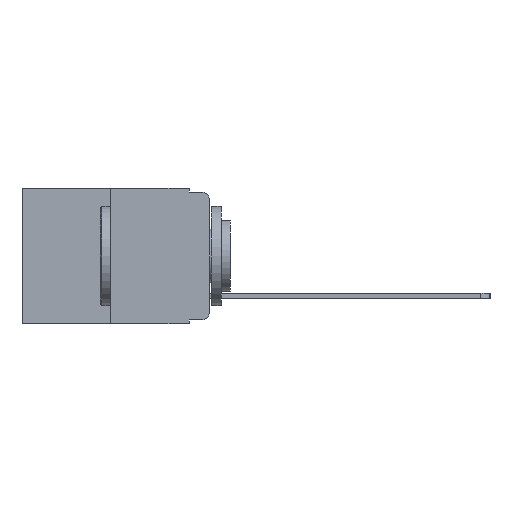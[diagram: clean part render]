
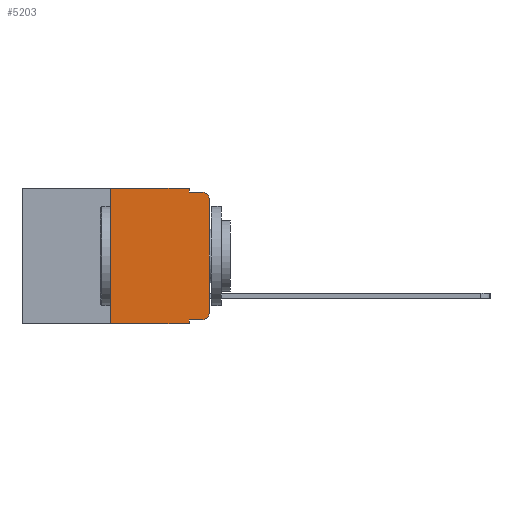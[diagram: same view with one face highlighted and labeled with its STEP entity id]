
A CAD part, left-side view. The second image highlights one B-rep face of the part: STEP entity #5203.
In plain terms, the highlighted planar face has unit normal (-1, 0, 0).
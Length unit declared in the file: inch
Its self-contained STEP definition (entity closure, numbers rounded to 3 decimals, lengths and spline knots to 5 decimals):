
#146 = LINE ( 'NONE', #504, #11594 ) ;
#258 = VERTEX_POINT ( 'NONE', #9818 ) ;
#504 = CARTESIAN_POINT ( 'NONE',  ( 0., 0., 0. ) ) ;
#538 = ORIENTED_EDGE ( 'NONE', *, *, #5592, .F. ) ;
#707 = ORIENTED_EDGE ( 'NONE', *, *, #5393, .F. ) ;
#801 = CARTESIAN_POINT ( 'NONE',  ( 0., 0.051, 0. ) ) ;
#826 = EDGE_CURVE ( 'NONE', #8402, #5616, #2717, .T. ) ;
#912 = ORIENTED_EDGE ( 'NONE', *, *, #3249, .F. ) ;
#1109 = VECTOR ( 'NONE', #1333, 39.37008 ) ;
#1115 = LINE ( 'NONE', #12775, #3952 ) ;
#1333 = DIRECTION ( 'NONE',  ( 0., 0., -1. ) ) ;
#1358 = CARTESIAN_POINT ( 'NONE',  ( 0., 0.051, 0. ) ) ;
#1480 = VERTEX_POINT ( 'NONE', #3114 ) ;
#1545 = VERTEX_POINT ( 'NONE', #9407 ) ;
#1655 = EDGE_CURVE ( 'NONE', #8402, #1545, #4308, .T. ) ;
#1674 = LINE ( 'NONE', #5324, #12825 ) ;
#1754 = ORIENTED_EDGE ( 'NONE', *, *, #10000, .T. ) ;
#1782 = ORIENTED_EDGE ( 'NONE', *, *, #9841, .T. ) ;
#1915 = ORIENTED_EDGE ( 'NONE', *, *, #7054, .T. ) ;
#2150 = CARTESIAN_POINT ( 'NONE',  ( 0., 0.051, 0. ) ) ;
#2279 = ORIENTED_EDGE ( 'NONE', *, *, #1655, .F. ) ;
#2567 = DIRECTION ( 'NONE',  ( -1., 0., 0. ) ) ;
#2634 = ORIENTED_EDGE ( 'NONE', *, *, #826, .T. ) ;
#2717 = LINE ( 'NONE', #13334, #13717 ) ;
#2757 = FACE_OUTER_BOUND ( 'NONE', #4951, .T. ) ;
#3110 = LINE ( 'NONE', #801, #14028 ) ;
#3114 = CARTESIAN_POINT ( 'NONE',  ( 0., 0.25, -0.343 ) ) ;
#3249 = EDGE_CURVE ( 'NONE', #1480, #258, #1674, .T. ) ;
#3304 = LINE ( 'NONE', #12474, #8816 ) ;
#3351 = ORIENTED_EDGE ( 'NONE', *, *, #13469, .T. ) ;
#3540 = DIRECTION ( 'NONE',  ( 0., 0., 1. ) ) ;
#3573 = DIRECTION ( 'NONE',  ( 0., -1., 0. ) ) ;
#3952 = VECTOR ( 'NONE', #10757, 39.37008 ) ;
#4308 = LINE ( 'NONE', #1358, #1109 ) ;
#4515 = DIRECTION ( 'NONE',  ( -1., 0., 0. ) ) ;
#4700 = AXIS2_PLACEMENT_3D ( 'NONE', #10874, #4515, #11909 ) ;
#4761 = DIRECTION ( 'NONE',  ( 0., 0., -1. ) ) ;
#4951 = EDGE_LOOP ( 'NONE', ( #1782, #1915, #12875, #538, #707, #912, #1754, #2279, #2634, #3351 ) ) ;
#5203 = ADVANCED_FACE ( 'NONE', ( #2757 ), #6976, .F. ) ;
#5254 = CARTESIAN_POINT ( 'NONE',  ( 0., 0., -0.03 ) ) ;
#5324 = CARTESIAN_POINT ( 'NONE',  ( 0., 0.25, 0. ) ) ;
#5393 = EDGE_CURVE ( 'NONE', #258, #11207, #3304, .T. ) ;
#5451 = VERTEX_POINT ( 'NONE', #5254 ) ;
#5592 = EDGE_CURVE ( 'NONE', #11207, #12204, #3110, .T. ) ;
#5616 = VERTEX_POINT ( 'NONE', #10762 ) ;
#5856 = DIRECTION ( 'NONE',  ( 0., -1., 0. ) ) ;
#6101 = CARTESIAN_POINT ( 'NONE',  ( 0., 0.02, -0.01 ) ) ;
#6353 = EDGE_CURVE ( 'NONE', #12204, #8382, #12911, .T. ) ;
#6976 = PLANE ( 'NONE',  #8974 ) ;
#7054 = EDGE_CURVE ( 'NONE', #5451, #8382, #8443, .T. ) ;
#7233 = CARTESIAN_POINT ( 'NONE',  ( 0., 0.051, -0.333 ) ) ;
#7377 = DIRECTION ( 'NONE',  ( 0., -1., 0. ) ) ;
#8036 = CARTESIAN_POINT ( 'NONE',  ( 0., 0.473, 0. ) ) ;
#8147 = CIRCLE ( 'NONE', #4700, 0.02 ) ;
#8382 = VERTEX_POINT ( 'NONE', #6101 ) ;
#8402 = VERTEX_POINT ( 'NONE', #7233 ) ;
#8443 = CIRCLE ( 'NONE', #12642, 0.02 ) ;
#8478 = CARTESIAN_POINT ( 'NONE',  ( 0., 0.051, -0.01 ) ) ;
#8816 = VECTOR ( 'NONE', #7377, 39.37008 ) ;
#8974 = AXIS2_PLACEMENT_3D ( 'NONE', #8036, #11059, #4761 ) ;
#9202 = CARTESIAN_POINT ( 'NONE',  ( 0., 0.02, -0.03 ) ) ;
#9407 = CARTESIAN_POINT ( 'NONE',  ( 0., 0.051, -0.343 ) ) ;
#9620 = VERTEX_POINT ( 'NONE', #12296 ) ;
#9794 = DIRECTION ( 'NONE',  ( 0., 0., -1. ) ) ;
#9818 = CARTESIAN_POINT ( 'NONE',  ( 0., 0.25, 0. ) ) ;
#9841 = EDGE_CURVE ( 'NONE', #9620, #5451, #146, .T. ) ;
#10000 = EDGE_CURVE ( 'NONE', #1480, #1545, #1115, .T. ) ;
#10210 = DIRECTION ( 'NONE',  ( 0., 0., -1. ) ) ;
#10229 = VECTOR ( 'NONE', #5856, 39.37008 ) ;
#10547 = DIRECTION ( 'NONE',  ( 0., 0., 1. ) ) ;
#10757 = DIRECTION ( 'NONE',  ( 0., -1., 0. ) ) ;
#10762 = CARTESIAN_POINT ( 'NONE',  ( 0., 0.02, -0.333 ) ) ;
#10874 = CARTESIAN_POINT ( 'NONE',  ( 0., 0.02, -0.313 ) ) ;
#11059 = DIRECTION ( 'NONE',  ( 1., 0., 0. ) ) ;
#11207 = VERTEX_POINT ( 'NONE', #2150 ) ;
#11594 = VECTOR ( 'NONE', #10547, 39.37008 ) ;
#11909 = DIRECTION ( 'NONE',  ( 0., 0., -1. ) ) ;
#12048 = CARTESIAN_POINT ( 'NONE',  ( 0., 0.051, -0.01 ) ) ;
#12204 = VERTEX_POINT ( 'NONE', #8478 ) ;
#12296 = CARTESIAN_POINT ( 'NONE',  ( 0., 0., -0.313 ) ) ;
#12474 = CARTESIAN_POINT ( 'NONE',  ( 0., 0.473, 0. ) ) ;
#12642 = AXIS2_PLACEMENT_3D ( 'NONE', #9202, #2567, #10210 ) ;
#12775 = CARTESIAN_POINT ( 'NONE',  ( 0., 0.473, -0.343 ) ) ;
#12825 = VECTOR ( 'NONE', #3540, 39.37008 ) ;
#12875 = ORIENTED_EDGE ( 'NONE', *, *, #6353, .F. ) ;
#12911 = LINE ( 'NONE', #12048, #10229 ) ;
#13334 = CARTESIAN_POINT ( 'NONE',  ( 0., 0.051, -0.333 ) ) ;
#13469 = EDGE_CURVE ( 'NONE', #5616, #9620, #8147, .T. ) ;
#13717 = VECTOR ( 'NONE', #3573, 39.37008 ) ;
#14028 = VECTOR ( 'NONE', #9794, 39.37008 ) ;
